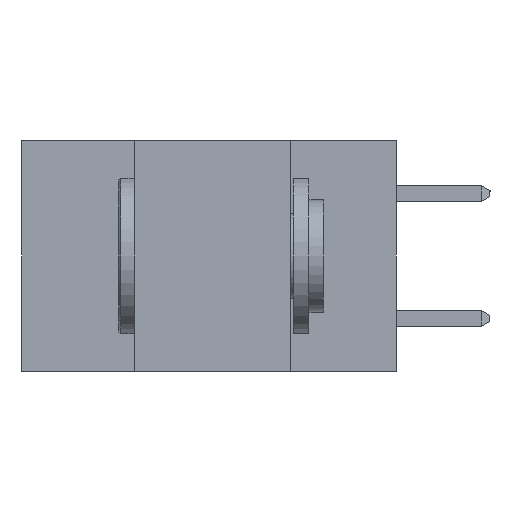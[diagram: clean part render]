
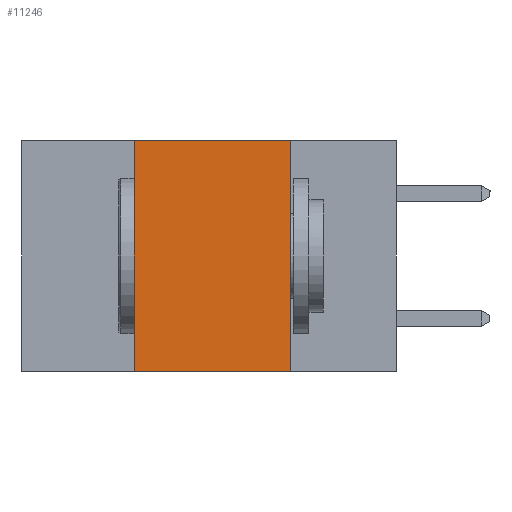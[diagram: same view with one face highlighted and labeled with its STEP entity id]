
A CAD part, left-side view. The second image highlights one B-rep face of the part: STEP entity #11246.
In plain terms, the highlighted planar face has unit normal (-1, 0, 0).
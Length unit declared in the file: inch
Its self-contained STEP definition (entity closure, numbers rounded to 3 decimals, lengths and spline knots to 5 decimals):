
#1091 = AXIS2_PLACEMENT_3D ( 'NONE', #10785, #4642, #9983 ) ;
#1210 = EDGE_CURVE ( 'NONE', #1990, #12412, #3414, .T. ) ;
#1990 = VERTEX_POINT ( 'NONE', #10586 ) ;
#2030 = CARTESIAN_POINT ( 'NONE',  ( 0., 0.17, -0.37 ) ) ;
#3084 = ORIENTED_EDGE ( 'NONE', *, *, #9950, .F. ) ;
#3414 = LINE ( 'NONE', #7207, #9224 ) ;
#4112 = DIRECTION ( 'NONE',  ( 0., 0., 1. ) ) ;
#4642 = DIRECTION ( 'NONE',  ( 1., 0., 0. ) ) ;
#4933 = DIRECTION ( 'NONE',  ( 0., 0., -1. ) ) ;
#5335 = VECTOR ( 'NONE', #4933, 39.37008 ) ;
#6513 = VECTOR ( 'NONE', #12899, 39.37008 ) ;
#7207 = CARTESIAN_POINT ( 'NONE',  ( 0., 0.6, 0. ) ) ;
#7583 = CARTESIAN_POINT ( 'NONE',  ( 0., 0.42, -0.37 ) ) ;
#7589 = CARTESIAN_POINT ( 'NONE',  ( 0., 0.42, -0.37 ) ) ;
#7948 = LINE ( 'NONE', #12741, #6513 ) ;
#8660 = DIRECTION ( 'NONE',  ( 0., -1., 0. ) ) ;
#9224 = VECTOR ( 'NONE', #8660, 39.37008 ) ;
#9631 = LINE ( 'NONE', #16019, #5335 ) ;
#9950 = EDGE_CURVE ( 'NONE', #12412, #12320, #9631, .T. ) ;
#9983 = DIRECTION ( 'NONE',  ( 0., 0., -1. ) ) ;
#10054 = EDGE_CURVE ( 'NONE', #13080, #1990, #13921, .T. ) ;
#10393 = ORIENTED_EDGE ( 'NONE', *, *, #1210, .F. ) ;
#10586 = CARTESIAN_POINT ( 'NONE',  ( 0., 0.42, 0. ) ) ;
#10785 = CARTESIAN_POINT ( 'NONE',  ( 0., 0.6, 0. ) ) ;
#11139 = EDGE_LOOP ( 'NONE', ( #3084, #10393, #12407, #15791 ) ) ;
#11246 = ADVANCED_FACE ( 'NONE', ( #12089 ), #14510, .F. ) ;
#12072 = VECTOR ( 'NONE', #4112, 39.37008 ) ;
#12089 = FACE_OUTER_BOUND ( 'NONE', #11139, .T. ) ;
#12320 = VERTEX_POINT ( 'NONE', #2030 ) ;
#12407 = ORIENTED_EDGE ( 'NONE', *, *, #10054, .F. ) ;
#12412 = VERTEX_POINT ( 'NONE', #14599 ) ;
#12741 = CARTESIAN_POINT ( 'NONE',  ( 0., 0.6, -0.37 ) ) ;
#12899 = DIRECTION ( 'NONE',  ( 0., -1., 0. ) ) ;
#13080 = VERTEX_POINT ( 'NONE', #7583 ) ;
#13921 = LINE ( 'NONE', #7589, #12072 ) ;
#14022 = EDGE_CURVE ( 'NONE', #13080, #12320, #7948, .T. ) ;
#14510 = PLANE ( 'NONE',  #1091 ) ;
#14599 = CARTESIAN_POINT ( 'NONE',  ( 0., 0.17, 0. ) ) ;
#15791 = ORIENTED_EDGE ( 'NONE', *, *, #14022, .T. ) ;
#16019 = CARTESIAN_POINT ( 'NONE',  ( 0., 0.17, -0.37 ) ) ;
